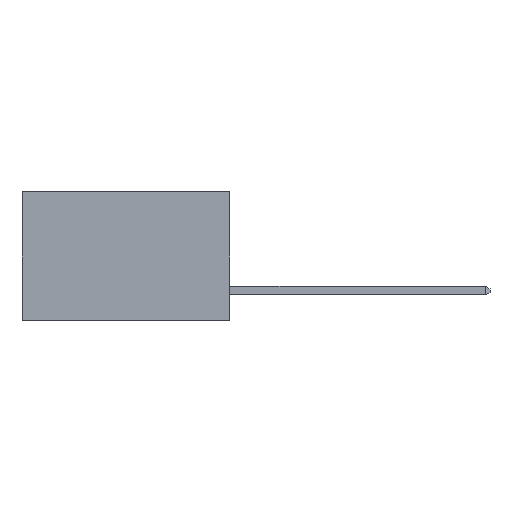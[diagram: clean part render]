
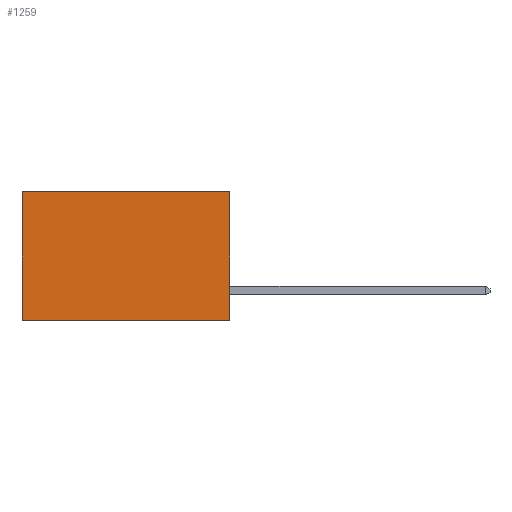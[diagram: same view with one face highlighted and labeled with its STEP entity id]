
A CAD part, left-side view. The second image highlights one B-rep face of the part: STEP entity #1259.
In plain terms, the highlighted planar face has unit normal (-1, 0, 0).
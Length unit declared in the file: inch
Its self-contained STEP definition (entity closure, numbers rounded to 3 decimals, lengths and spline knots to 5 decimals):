
#83 = CARTESIAN_POINT ( 'NONE',  ( 0.2615, 0., -0.37 ) ) ;
#365 = VECTOR ( 'NONE', #5332, 39.37008 ) ;
#612 = ORIENTED_EDGE ( 'NONE', *, *, #5354, .T. ) ;
#980 = VECTOR ( 'NONE', #5793, 39.37008 ) ;
#1259 = ADVANCED_FACE ( 'NONE', ( #6304 ), #6348, .F. ) ;
#1595 = EDGE_CURVE ( 'NONE', #1853, #6424, #2206, .T. ) ;
#1826 = ORIENTED_EDGE ( 'NONE', *, *, #2475, .T. ) ;
#1853 = VERTEX_POINT ( 'NONE', #6187 ) ;
#2159 = VECTOR ( 'NONE', #5001, 39.37008 ) ;
#2206 = LINE ( 'NONE', #7795, #365 ) ;
#2415 = VERTEX_POINT ( 'NONE', #6448 ) ;
#2475 = EDGE_CURVE ( 'NONE', #5057, #2415, #4449, .T. ) ;
#2933 = AXIS2_PLACEMENT_3D ( 'NONE', #6925, #5286, #4079 ) ;
#3814 = LINE ( 'NONE', #5024, #2159 ) ;
#4079 = DIRECTION ( 'NONE',  ( 0., 0., -1. ) ) ;
#4332 = DIRECTION ( 'NONE',  ( 0., 1., 0. ) ) ;
#4415 = CARTESIAN_POINT ( 'NONE',  ( 0.2615, 0., -0.37 ) ) ;
#4449 = LINE ( 'NONE', #5760, #980 ) ;
#5001 = DIRECTION ( 'NONE',  ( 0., 1., 0. ) ) ;
#5024 = CARTESIAN_POINT ( 'NONE',  ( 0.2615, 0., 0. ) ) ;
#5057 = VERTEX_POINT ( 'NONE', #6685 ) ;
#5069 = EDGE_LOOP ( 'NONE', ( #1826, #6843, #7003, #612 ) ) ;
#5286 = DIRECTION ( 'NONE',  ( 1., 0., 0. ) ) ;
#5332 = DIRECTION ( 'NONE',  ( 0., 0., -1. ) ) ;
#5354 = EDGE_CURVE ( 'NONE', #1853, #5057, #3814, .T. ) ;
#5445 = LINE ( 'NONE', #4415, #6764 ) ;
#5760 = CARTESIAN_POINT ( 'NONE',  ( 0.2615, 0.6, -0.37 ) ) ;
#5793 = DIRECTION ( 'NONE',  ( 0., 0., -1. ) ) ;
#6187 = CARTESIAN_POINT ( 'NONE',  ( 0.2615, 0., 0. ) ) ;
#6304 = FACE_OUTER_BOUND ( 'NONE', #5069, .T. ) ;
#6348 = PLANE ( 'NONE',  #2933 ) ;
#6424 = VERTEX_POINT ( 'NONE', #83 ) ;
#6448 = CARTESIAN_POINT ( 'NONE',  ( 0.2615, 0.6, -0.37 ) ) ;
#6685 = CARTESIAN_POINT ( 'NONE',  ( 0.2615, 0.6, 0. ) ) ;
#6764 = VECTOR ( 'NONE', #4332, 39.37008 ) ;
#6843 = ORIENTED_EDGE ( 'NONE', *, *, #7032, .F. ) ;
#6925 = CARTESIAN_POINT ( 'NONE',  ( 0.2615, 0., -0.37 ) ) ;
#7003 = ORIENTED_EDGE ( 'NONE', *, *, #1595, .F. ) ;
#7032 = EDGE_CURVE ( 'NONE', #6424, #2415, #5445, .T. ) ;
#7795 = CARTESIAN_POINT ( 'NONE',  ( 0.2615, 0., -0.37 ) ) ;
